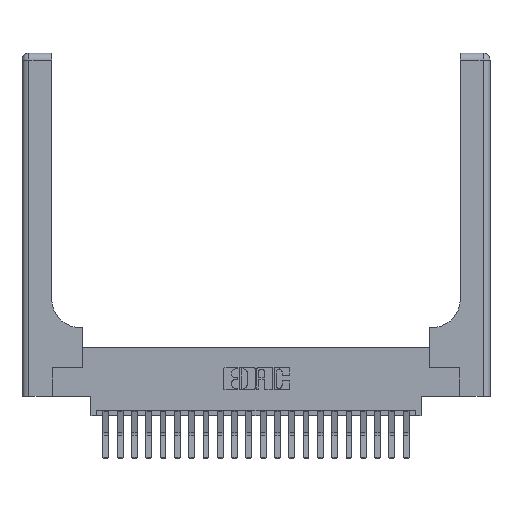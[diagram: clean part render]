
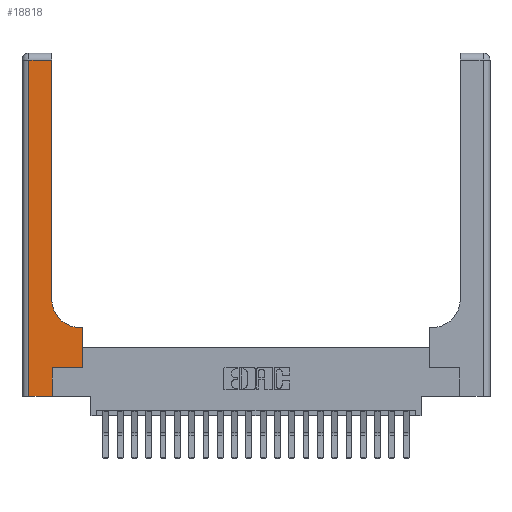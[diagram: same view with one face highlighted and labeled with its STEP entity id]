
A CAD part, top view. The second image highlights one B-rep face of the part: STEP entity #18818.
In plain terms, the highlighted planar face has unit normal (0, 0, 1).
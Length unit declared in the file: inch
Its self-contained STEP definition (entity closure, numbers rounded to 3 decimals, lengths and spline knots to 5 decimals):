
#45 = DIRECTION ( 'NONE',  ( -1., 0., 0. ) ) ;
#108 = CARTESIAN_POINT ( 'NONE',  ( 0.26, 0.85, 0.37 ) ) ;
#176 = ORIENTED_EDGE ( 'NONE', *, *, #20321, .T. ) ;
#382 = EDGE_CURVE ( 'NONE', #21398, #18540, #22563, .T. ) ;
#876 = CARTESIAN_POINT ( 'NONE',  ( 0.26, 3., 0.37 ) ) ;
#1057 = DIRECTION ( 'NONE',  ( 1., 0., 0. ) ) ;
#1194 = CARTESIAN_POINT ( 'NONE',  ( 0.265, 0., 0.37 ) ) ;
#1644 = EDGE_LOOP ( 'NONE', ( #10651, #10149, #3249, #17781, #5735, #10653, #2967, #16897, #176 ) ) ;
#1879 = DIRECTION ( 'NONE',  ( 0., 0., -1. ) ) ;
#2256 = VERTEX_POINT ( 'NONE', #13727 ) ;
#2564 = CARTESIAN_POINT ( 'NONE',  ( 0.265, 0., 0.37 ) ) ;
#2676 = CIRCLE ( 'NONE', #15284, 0.25 ) ;
#2695 = DIRECTION ( 'NONE',  ( 0., 0., -1. ) ) ;
#2967 = ORIENTED_EDGE ( 'NONE', *, *, #12871, .T. ) ;
#3249 = ORIENTED_EDGE ( 'NONE', *, *, #9689, .T. ) ;
#3391 = CARTESIAN_POINT ( 'NONE',  ( 0.528, 0.6, 0.37 ) ) ;
#3535 = VECTOR ( 'NONE', #15608, 39.37008 ) ;
#4080 = VERTEX_POINT ( 'NONE', #10465 ) ;
#4518 = DIRECTION ( 'NONE',  ( -1., 0., 0. ) ) ;
#4816 = CARTESIAN_POINT ( 'NONE',  ( 0., 2.94, 0.37 ) ) ;
#5129 = VERTEX_POINT ( 'NONE', #20586 ) ;
#5307 = VECTOR ( 'NONE', #4518, 39.37008 ) ;
#5466 = LINE ( 'NONE', #12316, #16372 ) ;
#5735 = ORIENTED_EDGE ( 'NONE', *, *, #17401, .T. ) ;
#6146 = VERTEX_POINT ( 'NONE', #2564 ) ;
#6224 = VECTOR ( 'NONE', #22329, 39.37008 ) ;
#6317 = LINE ( 'NONE', #1194, #20389 ) ;
#6337 = VERTEX_POINT ( 'NONE', #10103 ) ;
#6862 = DIRECTION ( 'NONE',  ( 0., -1., 0. ) ) ;
#7099 = EDGE_CURVE ( 'NONE', #12897, #6337, #8077, .T. ) ;
#8077 = LINE ( 'NONE', #876, #13060 ) ;
#9689 = EDGE_CURVE ( 'NONE', #4080, #5129, #22739, .T. ) ;
#9909 = DIRECTION ( 'NONE',  ( 0., 1., 0. ) ) ;
#9980 = CARTESIAN_POINT ( 'NONE',  ( 0.26, 0.6, 0.37 ) ) ;
#10103 = CARTESIAN_POINT ( 'NONE',  ( 0.26, 2.94, 0.37 ) ) ;
#10149 = ORIENTED_EDGE ( 'NONE', *, *, #11916, .T. ) ;
#10367 = VECTOR ( 'NONE', #19259, 39.37008 ) ;
#10465 = CARTESIAN_POINT ( 'NONE',  ( 0.06, 2.94, 0.37 ) ) ;
#10651 = ORIENTED_EDGE ( 'NONE', *, *, #7099, .T. ) ;
#10653 = ORIENTED_EDGE ( 'NONE', *, *, #382, .T. ) ;
#11916 = EDGE_CURVE ( 'NONE', #6337, #4080, #18860, .T. ) ;
#12120 = FACE_OUTER_BOUND ( 'NONE', #1644, .T. ) ;
#12187 = CARTESIAN_POINT ( 'NONE',  ( 0.528, 0.25, 0.37 ) ) ;
#12316 = CARTESIAN_POINT ( 'NONE',  ( 0., 0., 0.37 ) ) ;
#12339 = CARTESIAN_POINT ( 'NONE',  ( 0., 3., 0.37 ) ) ;
#12871 = EDGE_CURVE ( 'NONE', #18540, #20585, #15897, .T. ) ;
#12897 = VERTEX_POINT ( 'NONE', #108 ) ;
#13060 = VECTOR ( 'NONE', #18517, 39.37008 ) ;
#13727 = CARTESIAN_POINT ( 'NONE',  ( 0.51, 0.6, 0.37 ) ) ;
#13881 = CARTESIAN_POINT ( 'NONE',  ( 0.265, 0.25, 0.37 ) ) ;
#14048 = CARTESIAN_POINT ( 'NONE',  ( 0.06, 3., 0.37 ) ) ;
#14434 = CARTESIAN_POINT ( 'NONE',  ( 0.265, 0.25, 0.37 ) ) ;
#15106 = CARTESIAN_POINT ( 'NONE',  ( 0.51, 0.85, 0.37 ) ) ;
#15284 = AXIS2_PLACEMENT_3D ( 'NONE', #15106, #2695, #1057 ) ;
#15608 = DIRECTION ( 'NONE',  ( -1., 0., 0. ) ) ;
#15897 = LINE ( 'NONE', #12187, #10367 ) ;
#16372 = VECTOR ( 'NONE', #22743, 39.37008 ) ;
#16897 = ORIENTED_EDGE ( 'NONE', *, *, #20874, .T. ) ;
#17401 = EDGE_CURVE ( 'NONE', #6146, #21398, #6317, .T. ) ;
#17781 = ORIENTED_EDGE ( 'NONE', *, *, #19232, .T. ) ;
#18161 = CARTESIAN_POINT ( 'NONE',  ( 0.528, 0.25, 0.37 ) ) ;
#18517 = DIRECTION ( 'NONE',  ( 0., 1., 0. ) ) ;
#18540 = VERTEX_POINT ( 'NONE', #18161 ) ;
#18569 = AXIS2_PLACEMENT_3D ( 'NONE', #12339, #1879, #45 ) ;
#18818 = ADVANCED_FACE ( 'NONE', ( #12120 ), #20930, .F. ) ;
#18860 = LINE ( 'NONE', #4816, #3535 ) ;
#19232 = EDGE_CURVE ( 'NONE', #5129, #6146, #5466, .T. ) ;
#19259 = DIRECTION ( 'NONE',  ( 0., 1., 0. ) ) ;
#20321 = EDGE_CURVE ( 'NONE', #2256, #12897, #2676, .T. ) ;
#20389 = VECTOR ( 'NONE', #9909, 39.37008 ) ;
#20565 = VECTOR ( 'NONE', #6862, 39.37008 ) ;
#20585 = VERTEX_POINT ( 'NONE', #3391 ) ;
#20586 = CARTESIAN_POINT ( 'NONE',  ( 0.06, 0., 0.37 ) ) ;
#20874 = EDGE_CURVE ( 'NONE', #20585, #2256, #22260, .T. ) ;
#20930 = PLANE ( 'NONE',  #18569 ) ;
#21398 = VERTEX_POINT ( 'NONE', #14434 ) ;
#22260 = LINE ( 'NONE', #9980, #5307 ) ;
#22329 = DIRECTION ( 'NONE',  ( 1., 0., 0. ) ) ;
#22563 = LINE ( 'NONE', #13881, #6224 ) ;
#22739 = LINE ( 'NONE', #14048, #20565 ) ;
#22743 = DIRECTION ( 'NONE',  ( 1., 0., 0. ) ) ;
